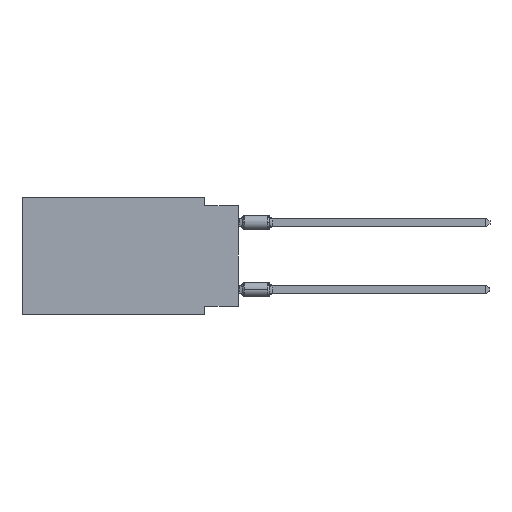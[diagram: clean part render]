
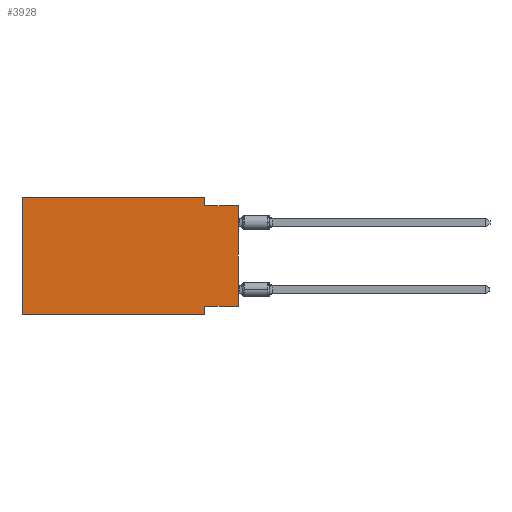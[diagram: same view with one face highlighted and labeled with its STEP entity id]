
A CAD part, left-side view. The second image highlights one B-rep face of the part: STEP entity #3928.
In plain terms, the highlighted planar face has unit normal (-1, 0, 0).
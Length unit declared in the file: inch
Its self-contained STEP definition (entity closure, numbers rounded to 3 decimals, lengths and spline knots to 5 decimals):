
#303 = CARTESIAN_POINT ( 'NONE',  ( 0., 0.1, -0.35 ) ) ;
#304 = VERTEX_POINT ( 'NONE', #12402 ) ;
#571 = CARTESIAN_POINT ( 'NONE',  ( 0., 0.1, -0.325 ) ) ;
#752 = EDGE_CURVE ( 'NONE', #15154, #3098, #16496, .T. ) ;
#1246 = VERTEX_POINT ( 'NONE', #15624 ) ;
#1830 = CARTESIAN_POINT ( 'NONE',  ( 0., 0., -0.025 ) ) ;
#2028 = ORIENTED_EDGE ( 'NONE', *, *, #13023, .F. ) ;
#2077 = DIRECTION ( 'NONE',  ( 0., -1., 0. ) ) ;
#3002 = DIRECTION ( 'NONE',  ( 0., -1., 0. ) ) ;
#3098 = VERTEX_POINT ( 'NONE', #9722 ) ;
#3223 = ORIENTED_EDGE ( 'NONE', *, *, #14030, .F. ) ;
#3303 = PLANE ( 'NONE',  #8815 ) ;
#3568 = CARTESIAN_POINT ( 'NONE',  ( 0., 0.645, 0. ) ) ;
#3591 = VECTOR ( 'NONE', #14332, 39.37008 ) ;
#3928 = ADVANCED_FACE ( 'NONE', ( #16297 ), #3303, .F. ) ;
#4151 = CARTESIAN_POINT ( 'NONE',  ( 0., 0.645, -0.35 ) ) ;
#4248 = EDGE_CURVE ( 'NONE', #15154, #1246, #15779, .T. ) ;
#4255 = CARTESIAN_POINT ( 'NONE',  ( 0., 0.1, 0. ) ) ;
#4413 = VECTOR ( 'NONE', #8158, 39.37008 ) ;
#4941 = DIRECTION ( 'NONE',  ( 0., 0., 1. ) ) ;
#5485 = VERTEX_POINT ( 'NONE', #571 ) ;
#5530 = VERTEX_POINT ( 'NONE', #12226 ) ;
#6246 = LINE ( 'NONE', #15492, #3591 ) ;
#6866 = LINE ( 'NONE', #303, #12098 ) ;
#7215 = LINE ( 'NONE', #1830, #13941 ) ;
#7940 = VECTOR ( 'NONE', #3002, 39.37008 ) ;
#8158 = DIRECTION ( 'NONE',  ( 0., 0., -1. ) ) ;
#8302 = ORIENTED_EDGE ( 'NONE', *, *, #10195, .F. ) ;
#8442 = ORIENTED_EDGE ( 'NONE', *, *, #12206, .F. ) ;
#8796 = VECTOR ( 'NONE', #9336, 39.37008 ) ;
#8815 = AXIS2_PLACEMENT_3D ( 'NONE', #12419, #13608, #11206 ) ;
#9223 = ORIENTED_EDGE ( 'NONE', *, *, #752, .F. ) ;
#9286 = VECTOR ( 'NONE', #15044, 39.37008 ) ;
#9336 = DIRECTION ( 'NONE',  ( 0., -1., 0. ) ) ;
#9360 = CARTESIAN_POINT ( 'NONE',  ( 0., 0.645, -0.35 ) ) ;
#9527 = EDGE_LOOP ( 'NONE', ( #9572, #8302, #12343, #3223, #9223, #14396, #8442, #2028 ) ) ;
#9572 = ORIENTED_EDGE ( 'NONE', *, *, #13822, .T. ) ;
#9722 = CARTESIAN_POINT ( 'NONE',  ( 0., 0.645, 0. ) ) ;
#10195 = EDGE_CURVE ( 'NONE', #5530, #14782, #7215, .T. ) ;
#10770 = DIRECTION ( 'NONE',  ( 0., 0., -1. ) ) ;
#11112 = LINE ( 'NONE', #16290, #9286 ) ;
#11206 = DIRECTION ( 'NONE',  ( 0., 0., -1. ) ) ;
#11585 = VECTOR ( 'NONE', #4941, 39.37008 ) ;
#11920 = CARTESIAN_POINT ( 'NONE',  ( 0., 0., -0.325 ) ) ;
#12098 = VECTOR ( 'NONE', #10770, 39.37008 ) ;
#12106 = LINE ( 'NONE', #14758, #7940 ) ;
#12206 = EDGE_CURVE ( 'NONE', #5485, #1246, #6866, .T. ) ;
#12226 = CARTESIAN_POINT ( 'NONE',  ( 0., 0.1, -0.025 ) ) ;
#12343 = ORIENTED_EDGE ( 'NONE', *, *, #13655, .F. ) ;
#12402 = CARTESIAN_POINT ( 'NONE',  ( 0., 0.1, 0. ) ) ;
#12419 = CARTESIAN_POINT ( 'NONE',  ( 0., 0.645, 0. ) ) ;
#12980 = VERTEX_POINT ( 'NONE', #11920 ) ;
#13023 = EDGE_CURVE ( 'NONE', #12980, #5485, #6246, .T. ) ;
#13336 = CARTESIAN_POINT ( 'NONE',  ( 0., 0., -0.025 ) ) ;
#13608 = DIRECTION ( 'NONE',  ( 1., 0., 0. ) ) ;
#13655 = EDGE_CURVE ( 'NONE', #304, #5530, #15882, .T. ) ;
#13822 = EDGE_CURVE ( 'NONE', #12980, #14782, #11112, .T. ) ;
#13941 = VECTOR ( 'NONE', #2077, 39.37008 ) ;
#14030 = EDGE_CURVE ( 'NONE', #3098, #304, #12106, .T. ) ;
#14332 = DIRECTION ( 'NONE',  ( 0., 1., 0. ) ) ;
#14396 = ORIENTED_EDGE ( 'NONE', *, *, #4248, .T. ) ;
#14758 = CARTESIAN_POINT ( 'NONE',  ( 0., 0.645, 0. ) ) ;
#14782 = VERTEX_POINT ( 'NONE', #13336 ) ;
#15044 = DIRECTION ( 'NONE',  ( 0., 0., 1. ) ) ;
#15154 = VERTEX_POINT ( 'NONE', #9360 ) ;
#15492 = CARTESIAN_POINT ( 'NONE',  ( 0., 0., -0.325 ) ) ;
#15624 = CARTESIAN_POINT ( 'NONE',  ( 0., 0.1, -0.35 ) ) ;
#15779 = LINE ( 'NONE', #4151, #8796 ) ;
#15882 = LINE ( 'NONE', #4255, #4413 ) ;
#16290 = CARTESIAN_POINT ( 'NONE',  ( 0., 0., 0. ) ) ;
#16297 = FACE_OUTER_BOUND ( 'NONE', #9527, .T. ) ;
#16496 = LINE ( 'NONE', #3568, #11585 ) ;
